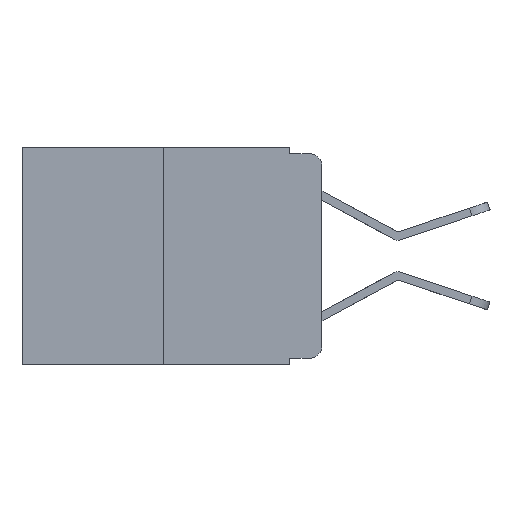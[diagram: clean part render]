
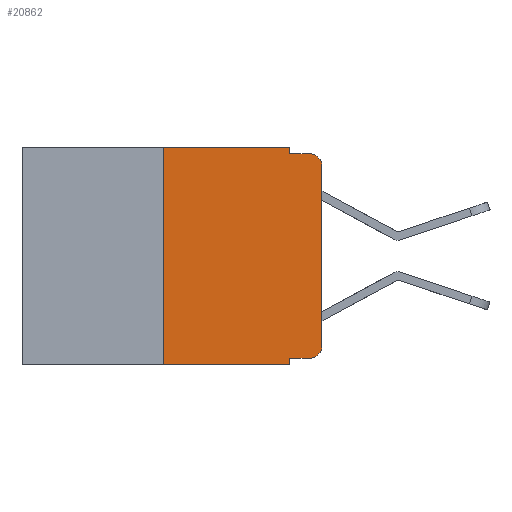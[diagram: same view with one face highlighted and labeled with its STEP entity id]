
A CAD part, left-side view. The second image highlights one B-rep face of the part: STEP entity #20862.
In plain terms, the highlighted planar face has unit normal (-1, 0, 0).
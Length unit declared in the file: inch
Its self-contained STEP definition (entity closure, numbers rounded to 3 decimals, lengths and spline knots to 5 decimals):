
#362 = CARTESIAN_POINT ( 'NONE',  ( 0., 0.051, 0. ) ) ;
#413 = VERTEX_POINT ( 'NONE', #18662 ) ;
#478 = VECTOR ( 'NONE', #14358, 39.37008 ) ;
#557 = AXIS2_PLACEMENT_3D ( 'NONE', #17136, #6404, #8023 ) ;
#629 = CARTESIAN_POINT ( 'NONE',  ( 0., 0.02, -0.333 ) ) ;
#813 = ORIENTED_EDGE ( 'NONE', *, *, #6205, .T. ) ;
#1125 = VECTOR ( 'NONE', #14682, 39.37008 ) ;
#1209 = FACE_OUTER_BOUND ( 'NONE', #5559, .T. ) ;
#1434 = EDGE_CURVE ( 'NONE', #20809, #9035, #6845, .T. ) ;
#1441 = ORIENTED_EDGE ( 'NONE', *, *, #6699, .T. ) ;
#1771 = DIRECTION ( 'NONE',  ( 0., 0., -1. ) ) ;
#1804 = AXIS2_PLACEMENT_3D ( 'NONE', #7363, #19810, #21577 ) ;
#2723 = LINE ( 'NONE', #12705, #478 ) ;
#3111 = ORIENTED_EDGE ( 'NONE', *, *, #8698, .F. ) ;
#3180 = EDGE_CURVE ( 'NONE', #20731, #21815, #3683, .T. ) ;
#3683 = LINE ( 'NONE', #17430, #14837 ) ;
#4169 = LINE ( 'NONE', #7590, #5298 ) ;
#4183 = AXIS2_PLACEMENT_3D ( 'NONE', #10413, #12427, #1771 ) ;
#4277 = ORIENTED_EDGE ( 'NONE', *, *, #8710, .F. ) ;
#4508 = PLANE ( 'NONE',  #557 ) ;
#5298 = VECTOR ( 'NONE', #21723, 39.37008 ) ;
#5416 = CARTESIAN_POINT ( 'NONE',  ( 0., 0., -0.03 ) ) ;
#5559 = EDGE_LOOP ( 'NONE', ( #1441, #20947, #5906, #3111, #6209, #20057, #22665, #4277, #813, #22705 ) ) ;
#5906 = ORIENTED_EDGE ( 'NONE', *, *, #9690, .F. ) ;
#6205 = EDGE_CURVE ( 'NONE', #16913, #20809, #7439, .T. ) ;
#6209 = ORIENTED_EDGE ( 'NONE', *, *, #9901, .F. ) ;
#6253 = DIRECTION ( 'NONE',  ( 0., 0., 1. ) ) ;
#6404 = DIRECTION ( 'NONE',  ( 1., 0., 0. ) ) ;
#6699 = EDGE_CURVE ( 'NONE', #9035, #15446, #18415, .T. ) ;
#6845 = CIRCLE ( 'NONE', #4183, 0.02 ) ;
#7168 = CARTESIAN_POINT ( 'NONE',  ( 0., 0.02, -0.01 ) ) ;
#7363 = CARTESIAN_POINT ( 'NONE',  ( 0., 0.02, -0.03 ) ) ;
#7439 = LINE ( 'NONE', #9976, #21089 ) ;
#7590 = CARTESIAN_POINT ( 'NONE',  ( 0., 0.051, 0. ) ) ;
#7993 = VERTEX_POINT ( 'NONE', #11859 ) ;
#8023 = DIRECTION ( 'NONE',  ( 0., 0., -1. ) ) ;
#8595 = VECTOR ( 'NONE', #16210, 39.37008 ) ;
#8698 = EDGE_CURVE ( 'NONE', #413, #18420, #4169, .T. ) ;
#8710 = EDGE_CURVE ( 'NONE', #16913, #7993, #11130, .T. ) ;
#8852 = VECTOR ( 'NONE', #9277, 39.37008 ) ;
#9035 = VERTEX_POINT ( 'NONE', #20379 ) ;
#9277 = DIRECTION ( 'NONE',  ( 0., -1., 0. ) ) ;
#9690 = EDGE_CURVE ( 'NONE', #18420, #22328, #19716, .T. ) ;
#9901 = EDGE_CURVE ( 'NONE', #21815, #413, #12447, .T. ) ;
#9976 = CARTESIAN_POINT ( 'NONE',  ( 0., 0.051, -0.333 ) ) ;
#10083 = CARTESIAN_POINT ( 'NONE',  ( 0., 0.051, -0.01 ) ) ;
#10273 = EDGE_CURVE ( 'NONE', #20731, #7993, #2723, .T. ) ;
#10413 = CARTESIAN_POINT ( 'NONE',  ( 0., 0.02, -0.313 ) ) ;
#10481 = VECTOR ( 'NONE', #6253, 39.37008 ) ;
#11118 = CARTESIAN_POINT ( 'NONE',  ( 0., 0.473, 0. ) ) ;
#11130 = LINE ( 'NONE', #362, #1125 ) ;
#11859 = CARTESIAN_POINT ( 'NONE',  ( 0., 0.051, -0.343 ) ) ;
#12427 = DIRECTION ( 'NONE',  ( -1., 0., 0. ) ) ;
#12447 = LINE ( 'NONE', #11118, #8852 ) ;
#12449 = EDGE_CURVE ( 'NONE', #15446, #22328, #17926, .T. ) ;
#12705 = CARTESIAN_POINT ( 'NONE',  ( 0., 0.473, -0.343 ) ) ;
#12787 = CARTESIAN_POINT ( 'NONE',  ( 0., 0.25, 0. ) ) ;
#13146 = CARTESIAN_POINT ( 'NONE',  ( 0., 0., 0. ) ) ;
#14358 = DIRECTION ( 'NONE',  ( 0., -1., 0. ) ) ;
#14682 = DIRECTION ( 'NONE',  ( 0., 0., -1. ) ) ;
#14793 = CARTESIAN_POINT ( 'NONE',  ( 0., 0.25, -0.343 ) ) ;
#14837 = VECTOR ( 'NONE', #15793, 39.37008 ) ;
#15446 = VERTEX_POINT ( 'NONE', #5416 ) ;
#15756 = DIRECTION ( 'NONE',  ( 0., -1., 0. ) ) ;
#15793 = DIRECTION ( 'NONE',  ( 0., 0., 1. ) ) ;
#16210 = DIRECTION ( 'NONE',  ( 0., -1., 0. ) ) ;
#16288 = CARTESIAN_POINT ( 'NONE',  ( 0., 0.051, -0.01 ) ) ;
#16913 = VERTEX_POINT ( 'NONE', #20679 ) ;
#17136 = CARTESIAN_POINT ( 'NONE',  ( 0., 0.473, 0. ) ) ;
#17430 = CARTESIAN_POINT ( 'NONE',  ( 0., 0.25, 0. ) ) ;
#17926 = CIRCLE ( 'NONE', #1804, 0.02 ) ;
#18415 = LINE ( 'NONE', #13146, #10481 ) ;
#18420 = VERTEX_POINT ( 'NONE', #10083 ) ;
#18662 = CARTESIAN_POINT ( 'NONE',  ( 0., 0.051, 0. ) ) ;
#19716 = LINE ( 'NONE', #16288, #8595 ) ;
#19810 = DIRECTION ( 'NONE',  ( -1., 0., 0. ) ) ;
#20057 = ORIENTED_EDGE ( 'NONE', *, *, #3180, .F. ) ;
#20379 = CARTESIAN_POINT ( 'NONE',  ( 0., 0., -0.313 ) ) ;
#20679 = CARTESIAN_POINT ( 'NONE',  ( 0., 0.051, -0.333 ) ) ;
#20731 = VERTEX_POINT ( 'NONE', #14793 ) ;
#20809 = VERTEX_POINT ( 'NONE', #629 ) ;
#20862 = ADVANCED_FACE ( 'NONE', ( #1209 ), #4508, .F. ) ;
#20947 = ORIENTED_EDGE ( 'NONE', *, *, #12449, .T. ) ;
#21089 = VECTOR ( 'NONE', #15756, 39.37008 ) ;
#21577 = DIRECTION ( 'NONE',  ( 0., 0., -1. ) ) ;
#21723 = DIRECTION ( 'NONE',  ( 0., 0., -1. ) ) ;
#21815 = VERTEX_POINT ( 'NONE', #12787 ) ;
#22328 = VERTEX_POINT ( 'NONE', #7168 ) ;
#22665 = ORIENTED_EDGE ( 'NONE', *, *, #10273, .T. ) ;
#22705 = ORIENTED_EDGE ( 'NONE', *, *, #1434, .T. ) ;
